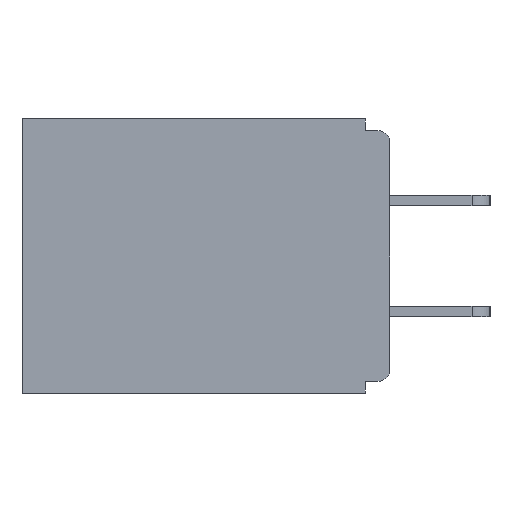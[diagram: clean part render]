
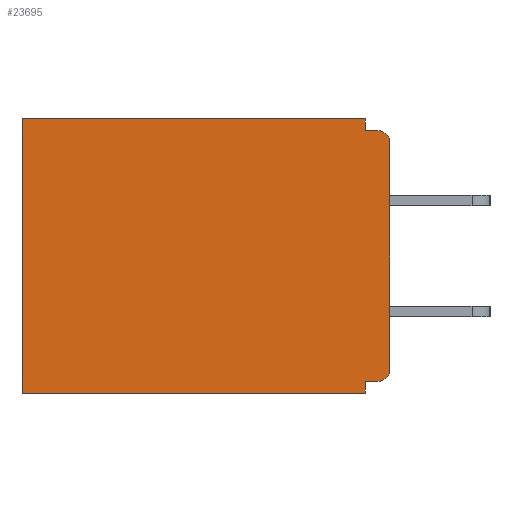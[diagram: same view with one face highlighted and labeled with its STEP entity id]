
A CAD part, left-side view. The second image highlights one B-rep face of the part: STEP entity #23695.
In plain terms, the highlighted planar face has unit normal (-1, 0, 0).
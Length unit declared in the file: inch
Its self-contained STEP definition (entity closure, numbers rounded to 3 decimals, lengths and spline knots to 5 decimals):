
#276 = AXIS2_PLACEMENT_3D ( 'NONE', #10639, #15365, #10332 ) ;
#599 = ORIENTED_EDGE ( 'NONE', *, *, #22412, .F. ) ;
#1261 = DIRECTION ( 'NONE',  ( 0., 0., -1. ) ) ;
#1360 = ORIENTED_EDGE ( 'NONE', *, *, #20619, .T. ) ;
#1367 = CARTESIAN_POINT ( 'NONE',  ( 0.298, 0.46, -0.343 ) ) ;
#2613 = ORIENTED_EDGE ( 'NONE', *, *, #27206, .F. ) ;
#2894 = VECTOR ( 'NONE', #16448, 39.37008 ) ;
#2965 = LINE ( 'NONE', #18015, #14074 ) ;
#3212 = EDGE_CURVE ( 'NONE', #16615, #24615, #9211, .T. ) ;
#3487 = PLANE ( 'NONE',  #276 ) ;
#3699 = VECTOR ( 'NONE', #26267, 39.37008 ) ;
#4593 = DIRECTION ( 'NONE',  ( 0., 0., -1. ) ) ;
#4802 = VECTOR ( 'NONE', #25758, 39.37008 ) ;
#5197 = VERTEX_POINT ( 'NONE', #20985 ) ;
#5256 = VERTEX_POINT ( 'NONE', #26253 ) ;
#5485 = CARTESIAN_POINT ( 'NONE',  ( 0.298, 0., -0.328 ) ) ;
#5694 = DIRECTION ( 'NONE',  ( -1., 0., 0. ) ) ;
#6119 = EDGE_CURVE ( 'NONE', #14437, #7124, #23365, .T. ) ;
#6377 = LINE ( 'NONE', #5485, #20071 ) ;
#6615 = CIRCLE ( 'NONE', #15747, 0.015 ) ;
#6931 = CARTESIAN_POINT ( 'NONE',  ( 0.298, 0., -0.015 ) ) ;
#7118 = CARTESIAN_POINT ( 'NONE',  ( 0.298, 0., 0. ) ) ;
#7124 = VERTEX_POINT ( 'NONE', #25133 ) ;
#7752 = LINE ( 'NONE', #20709, #10914 ) ;
#7859 = CARTESIAN_POINT ( 'NONE',  ( 0.298, 0.015, -0.313 ) ) ;
#8263 = VERTEX_POINT ( 'NONE', #22616 ) ;
#8739 = FACE_OUTER_BOUND ( 'NONE', #29859, .T. ) ;
#8914 = CARTESIAN_POINT ( 'NONE',  ( 0.298, 0.46, 0. ) ) ;
#9211 = LINE ( 'NONE', #6931, #2894 ) ;
#10058 = CARTESIAN_POINT ( 'NONE',  ( 0.298, 0.015, -0.03 ) ) ;
#10314 = VERTEX_POINT ( 'NONE', #28398 ) ;
#10332 = DIRECTION ( 'NONE',  ( 0., 0., -1. ) ) ;
#10639 = CARTESIAN_POINT ( 'NONE',  ( 0.298, 0., 0. ) ) ;
#10914 = VECTOR ( 'NONE', #13846, 39.37008 ) ;
#11311 = ORIENTED_EDGE ( 'NONE', *, *, #26465, .F. ) ;
#11561 = CARTESIAN_POINT ( 'NONE',  ( 0.298, 0.031, -0.015 ) ) ;
#11758 = CARTESIAN_POINT ( 'NONE',  ( 0.298, 0.031, -0.343 ) ) ;
#12672 = AXIS2_PLACEMENT_3D ( 'NONE', #7859, #5694, #21952 ) ;
#12979 = CARTESIAN_POINT ( 'NONE',  ( 0.298, 0.015, -0.015 ) ) ;
#13390 = VERTEX_POINT ( 'NONE', #26301 ) ;
#13535 = EDGE_CURVE ( 'NONE', #5256, #24571, #7752, .T. ) ;
#13846 = DIRECTION ( 'NONE',  ( 0., 1., 0. ) ) ;
#13937 = EDGE_CURVE ( 'NONE', #5197, #24615, #6615, .T. ) ;
#14074 = VECTOR ( 'NONE', #1261, 39.37008 ) ;
#14437 = VERTEX_POINT ( 'NONE', #27803 ) ;
#14680 = DIRECTION ( 'NONE',  ( 0., 0., -1. ) ) ;
#15365 = DIRECTION ( 'NONE',  ( 1., 0., 0. ) ) ;
#15717 = DIRECTION ( 'NONE',  ( 0., 0., -1. ) ) ;
#15747 = AXIS2_PLACEMENT_3D ( 'NONE', #10058, #22159, #14680 ) ;
#16054 = ORIENTED_EDGE ( 'NONE', *, *, #13535, .F. ) ;
#16410 = CARTESIAN_POINT ( 'NONE',  ( 0.298, 0.031, -0.343 ) ) ;
#16448 = DIRECTION ( 'NONE',  ( 0., -1., 0. ) ) ;
#16615 = VERTEX_POINT ( 'NONE', #11561 ) ;
#16655 = ORIENTED_EDGE ( 'NONE', *, *, #18607, .T. ) ;
#16852 = ORIENTED_EDGE ( 'NONE', *, *, #27889, .F. ) ;
#17216 = CIRCLE ( 'NONE', #12672, 0.015 ) ;
#18015 = CARTESIAN_POINT ( 'NONE',  ( 0.298, 0., 0. ) ) ;
#18607 = EDGE_CURVE ( 'NONE', #10314, #8263, #17216, .T. ) ;
#18837 = VECTOR ( 'NONE', #4593, 39.37008 ) ;
#19923 = ORIENTED_EDGE ( 'NONE', *, *, #3212, .F. ) ;
#19975 = LINE ( 'NONE', #16410, #18837 ) ;
#20071 = VECTOR ( 'NONE', #24746, 39.37008 ) ;
#20619 = EDGE_CURVE ( 'NONE', #7124, #24571, #29734, .T. ) ;
#20709 = CARTESIAN_POINT ( 'NONE',  ( 0.298, 0., -0.343 ) ) ;
#20897 = ORIENTED_EDGE ( 'NONE', *, *, #6119, .T. ) ;
#20985 = CARTESIAN_POINT ( 'NONE',  ( 0.298, 0., -0.03 ) ) ;
#21952 = DIRECTION ( 'NONE',  ( 0., 0., -1. ) ) ;
#22159 = DIRECTION ( 'NONE',  ( -1., 0., 0. ) ) ;
#22412 = EDGE_CURVE ( 'NONE', #14437, #16615, #28514, .T. ) ;
#22616 = CARTESIAN_POINT ( 'NONE',  ( 0.298, 0., -0.313 ) ) ;
#23365 = LINE ( 'NONE', #7118, #3699 ) ;
#23472 = VECTOR ( 'NONE', #15717, 39.37008 ) ;
#23695 = ADVANCED_FACE ( 'NONE', ( #8739 ), #3487, .F. ) ;
#24571 = VERTEX_POINT ( 'NONE', #1367 ) ;
#24615 = VERTEX_POINT ( 'NONE', #12979 ) ;
#24746 = DIRECTION ( 'NONE',  ( 0., 1., 0. ) ) ;
#25133 = CARTESIAN_POINT ( 'NONE',  ( 0.298, 0.46, 0. ) ) ;
#25758 = DIRECTION ( 'NONE',  ( 0., 0., -1. ) ) ;
#26253 = CARTESIAN_POINT ( 'NONE',  ( 0.298, 0.031, -0.343 ) ) ;
#26267 = DIRECTION ( 'NONE',  ( 0., 1., 0. ) ) ;
#26301 = CARTESIAN_POINT ( 'NONE',  ( 0.298, 0.031, -0.328 ) ) ;
#26465 = EDGE_CURVE ( 'NONE', #10314, #13390, #6377, .T. ) ;
#26638 = ORIENTED_EDGE ( 'NONE', *, *, #13937, .T. ) ;
#27206 = EDGE_CURVE ( 'NONE', #5197, #8263, #2965, .T. ) ;
#27803 = CARTESIAN_POINT ( 'NONE',  ( 0.298, 0.031, 0. ) ) ;
#27889 = EDGE_CURVE ( 'NONE', #13390, #5256, #19975, .T. ) ;
#28398 = CARTESIAN_POINT ( 'NONE',  ( 0.298, 0.015, -0.328 ) ) ;
#28514 = LINE ( 'NONE', #11758, #4802 ) ;
#29734 = LINE ( 'NONE', #8914, #23472 ) ;
#29859 = EDGE_LOOP ( 'NONE', ( #26638, #19923, #599, #20897, #1360, #16054, #16852, #11311, #16655, #2613 ) ) ;
